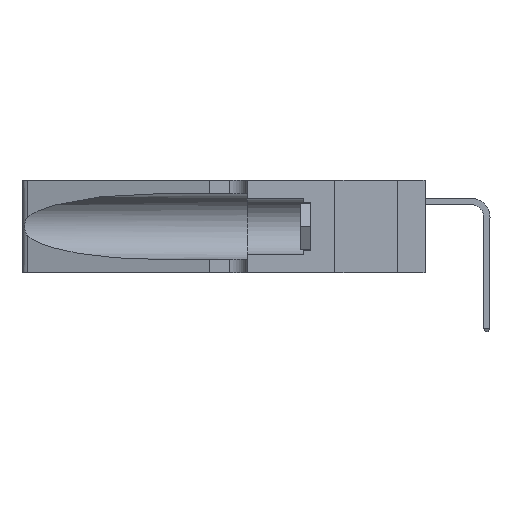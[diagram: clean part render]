
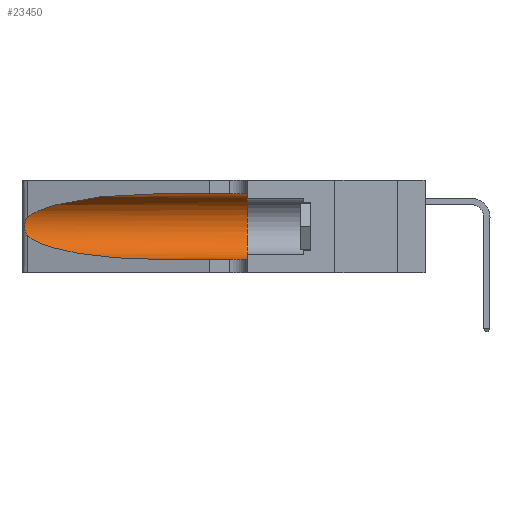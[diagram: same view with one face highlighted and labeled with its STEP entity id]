
A CAD part, left-side view. The second image highlights one B-rep face of the part: STEP entity #23450.
In plain terms, the highlighted cylindrical face has radius 3.308 mm (diameter 6.617 mm), a partial arc.
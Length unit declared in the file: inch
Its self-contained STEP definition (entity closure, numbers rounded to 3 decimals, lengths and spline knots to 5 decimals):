
#181 = VERTEX_POINT ( 'NONE', #8025 ) ;
#405 = CARTESIAN_POINT ( 'NONE',  ( 0.2373, 1.15595, 0.08982 ) ) ;
#547 = CARTESIAN_POINT ( 'NONE',  ( 0.25487, 1.22718, 0.22369 ) ) ;
#596 = LINE ( 'NONE', #2660, #6685 ) ;
#722 = CARTESIAN_POINT ( 'NONE',  ( 0.1305, 0.72297, 0.05475 ) ) ;
#1239 = VERTEX_POINT ( 'NONE', #13470 ) ;
#1676 = CARTESIAN_POINT ( 'NONE',  ( 0.26075, 1.23896, 0.19203 ) ) ;
#1845 = VERTEX_POINT ( 'NONE', #12033 ) ;
#2660 = CARTESIAN_POINT ( 'NONE',  ( 0.1305, 1.61858, 0.31525 ) ) ;
#2760 = VERTEX_POINT ( 'NONE', #17106 ) ;
#2868 = ORIENTED_EDGE ( 'NONE', *, *, #12155, .T. ) ;
#2926 = VERTEX_POINT ( 'NONE', #26378 ) ;
#3245 = ORIENTED_EDGE ( 'NONE', *, *, #25677, .T. ) ;
#3612 = CARTESIAN_POINT ( 'NONE',  ( 0.1305, 1.61858, 0.185 ) ) ;
#4018 = CARTESIAN_POINT ( 'NONE',  ( 0.26017, 1.23833, 0.17102 ) ) ;
#4708 = VECTOR ( 'NONE', #28268, 39.37008 ) ;
#5414 = EDGE_CURVE ( 'NONE', #15478, #1845, #20068, .T. ) ;
#6290 = CARTESIAN_POINT ( 'NONE',  ( 0.25789, 1.23486, 0.15765 ) ) ;
#6685 = VECTOR ( 'NONE', #22287, 39.37008 ) ;
#6927 = AXIS2_PLACEMENT_3D ( 'NONE', #3612, #18951, #12412 ) ;
#7464 = EDGE_CURVE ( 'NONE', #1239, #181, #596, .T. ) ;
#7551 = ORIENTED_EDGE ( 'NONE', *, *, #23193, .T. ) ;
#8025 = CARTESIAN_POINT ( 'NONE',  ( 0.1305, 0.35, 0.31525 ) ) ;
#8507 = CARTESIAN_POINT ( 'NONE',  ( 0.25555, 1.22993, 0.14849 ) ) ;
#9900 = ORIENTED_EDGE ( 'NONE', *, *, #11286, .F. ) ;
#11286 = EDGE_CURVE ( 'NONE', #181, #1845, #26287, .T. ) ;
#11718 = CARTESIAN_POINT ( 'NONE',  ( 0.18966, 0.96281, 0.31525 ) ) ;
#12033 = CARTESIAN_POINT ( 'NONE',  ( 0.1305, 0.35, 0.05475 ) ) ;
#12155 = EDGE_CURVE ( 'NONE', #1239, #2760, #24571, .T. ) ;
#12412 = DIRECTION ( 'NONE',  ( 0., 0., -1. ) ) ;
#12790 = CARTESIAN_POINT ( 'NONE',  ( 0.25787, 1.23484, 0.2124 ) ) ;
#13269 = DIRECTION ( 'NONE',  ( 0., 1., 0. ) ) ;
#13470 = CARTESIAN_POINT ( 'NONE',  ( 0.1305, 0.72297, 0.31525 ) ) ;
#13851 = CARTESIAN_POINT ( 'NONE',  ( 0.1305, 0.72297, 0.05475 ) ) ;
#13898 = CARTESIAN_POINT ( 'NONE',  ( 0.2373, 1.15595, 0.28018 ) ) ;
#14975 = CARTESIAN_POINT ( 'NONE',  ( 0.26018, 1.23835, 0.19895 ) ) ;
#15277 = FACE_OUTER_BOUND ( 'NONE', #20102, .T. ) ;
#15478 = VERTEX_POINT ( 'NONE', #722 ) ;
#16561 =( BOUNDED_CURVE ( )  B_SPLINE_CURVE ( 3, ( #18122, #405, #26805, #13851 ),
 .UNSPECIFIED., .F., .F. ) 
 B_SPLINE_CURVE_WITH_KNOTS ( ( 4, 4 ),
 ( 3.44316, 4.71239 ),
 .UNSPECIFIED. ) 
 CURVE ( )  GEOMETRIC_REPRESENTATION_ITEM ( )  RATIONAL_B_SPLINE_CURVE ( ( 1., 0.87, 0.87, 1. ) ) 
 REPRESENTATION_ITEM ( '' )  );
#16657 = ORIENTED_EDGE ( 'NONE', *, *, #7464, .F. ) ;
#17106 = CARTESIAN_POINT ( 'NONE',  ( 0.25487, 1.22718, 0.22369 ) ) ;
#17151 = CARTESIAN_POINT ( 'NONE',  ( 0.26075, 1.23896, 0.178 ) ) ;
#18122 = CARTESIAN_POINT ( 'NONE',  ( 0.25487, 1.22718, 0.14631 ) ) ;
#18951 = DIRECTION ( 'NONE',  ( 0., -1., 0. ) ) ;
#19337 = CARTESIAN_POINT ( 'NONE',  ( 0.25856, 1.23593, 0.16098 ) ) ;
#20068 = LINE ( 'NONE', #26210, #4708 ) ;
#20077 = ORIENTED_EDGE ( 'NONE', *, *, #5414, .T. ) ;
#20102 = EDGE_LOOP ( 'NONE', ( #2868, #3245, #7551, #20077, #9900, #16657 ) ) ;
#21385 = CARTESIAN_POINT ( 'NONE',  ( 0.25487, 1.22718, 0.22369 ) ) ;
#21483 = CARTESIAN_POINT ( 'NONE',  ( 0.25639, 1.23186, 0.15144 ) ) ;
#22287 = DIRECTION ( 'NONE',  ( 0., -1., 0. ) ) ;
#23193 = EDGE_CURVE ( 'NONE', #2926, #15478, #16561, .T. ) ;
#23450 = ADVANCED_FACE ( 'NONE', ( #15277 ), #26114, .F. ) ;
#23598 = CARTESIAN_POINT ( 'NONE',  ( 0.25555, 1.22994, 0.2215 ) ) ;
#23691 = CARTESIAN_POINT ( 'NONE',  ( 0.25487, 1.22718, 0.14631 ) ) ;
#24571 =( BOUNDED_CURVE ( )  B_SPLINE_CURVE ( 3, ( #24713, #11718, #13898, #547 ),
 .UNSPECIFIED., .F., .T. ) 
 B_SPLINE_CURVE_WITH_KNOTS ( ( 4, 4 ),
 ( 1.5708, 2.84003 ),
 .UNSPECIFIED. ) 
 CURVE ( )  GEOMETRIC_REPRESENTATION_ITEM ( )  RATIONAL_B_SPLINE_CURVE ( ( 1., 0.87, 0.87, 1. ) ) 
 REPRESENTATION_ITEM ( '' )  );
#24713 = CARTESIAN_POINT ( 'NONE',  ( 0.1305, 0.72297, 0.31525 ) ) ;
#25677 = EDGE_CURVE ( 'NONE', #2760, #2926, #26632, .T. ) ;
#25770 = CARTESIAN_POINT ( 'NONE',  ( 0.25639, 1.23184, 0.21858 ) ) ;
#26114 = CYLINDRICAL_SURFACE ( 'NONE', #6927, 0.13025 ) ;
#26210 = CARTESIAN_POINT ( 'NONE',  ( 0.1305, 1.61858, 0.05475 ) ) ;
#26246 = CARTESIAN_POINT ( 'NONE',  ( 0.1305, 0.35, 0.185 ) ) ;
#26287 = CIRCLE ( 'NONE', #28433, 0.13025 ) ;
#26378 = CARTESIAN_POINT ( 'NONE',  ( 0.25487, 1.22718, 0.14631 ) ) ;
#26632 = B_SPLINE_CURVE_WITH_KNOTS ( 'NONE', 3,
 ( #21385, #23598, #25770, #12790, #27907, #14975, #1676, #17151, #4018, #19337, #6290, #21483, #8507, #23691 ),
 .UNSPECIFIED., .F., .F.,
 ( 4, 2, 2, 2, 2, 2, 4 ),
 ( 0., 0.00027, 0.00053, 0.00107, 0.0016, 0.00187, 0.00214 ),
 .UNSPECIFIED. ) ;
#26805 = CARTESIAN_POINT ( 'NONE',  ( 0.18966, 0.96281, 0.05475 ) ) ;
#27907 = CARTESIAN_POINT ( 'NONE',  ( 0.25854, 1.2359, 0.20912 ) ) ;
#28268 = DIRECTION ( 'NONE',  ( 0., -1., 0. ) ) ;
#28404 = DIRECTION ( 'NONE',  ( 0., 0., 1. ) ) ;
#28433 = AXIS2_PLACEMENT_3D ( 'NONE', #26246, #13269, #28404 ) ;
